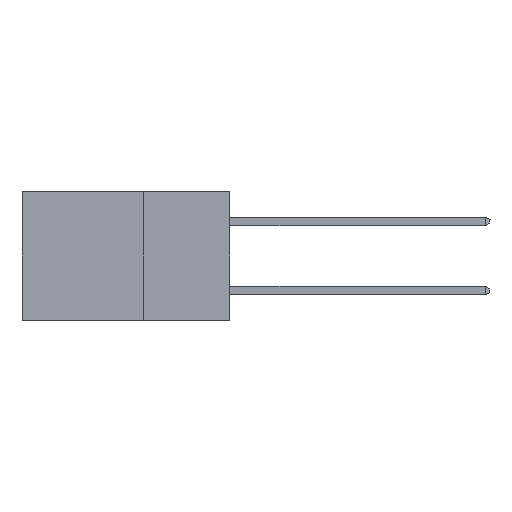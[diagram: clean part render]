
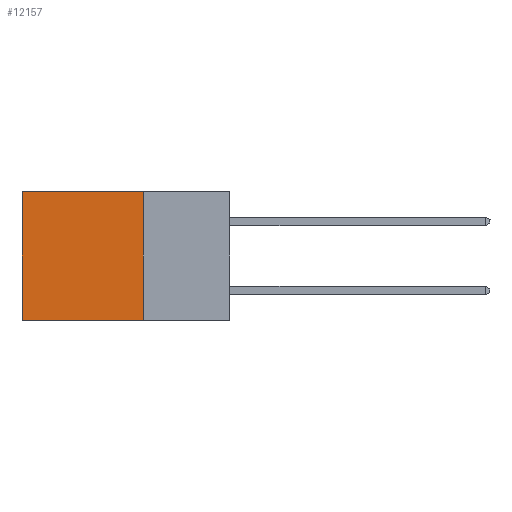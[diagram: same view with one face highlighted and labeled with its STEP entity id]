
A CAD part, left-side view. The second image highlights one B-rep face of the part: STEP entity #12157.
In plain terms, the highlighted planar face has unit normal (-1, 0, 0).
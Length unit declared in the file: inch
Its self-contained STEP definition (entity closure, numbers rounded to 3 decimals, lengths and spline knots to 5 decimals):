
#2193 = FACE_OUTER_BOUND ( 'NONE', #27637, .T. ) ;
#2243 = PLANE ( 'NONE',  #32307 ) ;
#2352 = LINE ( 'NONE', #3856, #28140 ) ;
#2664 = ORIENTED_EDGE ( 'NONE', *, *, #21250, .T. ) ;
#3313 = CARTESIAN_POINT ( 'NONE',  ( 0.298, 0.25, 0. ) ) ;
#3856 = CARTESIAN_POINT ( 'NONE',  ( 0.298, 0.25, 0. ) ) ;
#5920 = LINE ( 'NONE', #29463, #21591 ) ;
#7226 = CARTESIAN_POINT ( 'NONE',  ( 0.298, 0.25, -0.37 ) ) ;
#7919 = EDGE_CURVE ( 'NONE', #17606, #12598, #22392, .T. ) ;
#9897 = EDGE_CURVE ( 'NONE', #25952, #10006, #29351, .T. ) ;
#9940 = EDGE_CURVE ( 'NONE', #25952, #17606, #2352, .T. ) ;
#10006 = VERTEX_POINT ( 'NONE', #13774 ) ;
#12157 = ADVANCED_FACE ( 'NONE', ( #2193 ), #2243, .F. ) ;
#12348 = DIRECTION ( 'NONE',  ( 0., 0., -1. ) ) ;
#12598 = VERTEX_POINT ( 'NONE', #27733 ) ;
#13774 = CARTESIAN_POINT ( 'NONE',  ( 0.298, 0.6, 0. ) ) ;
#14659 = ORIENTED_EDGE ( 'NONE', *, *, #9940, .F. ) ;
#15110 = ORIENTED_EDGE ( 'NONE', *, *, #9897, .T. ) ;
#15202 = VECTOR ( 'NONE', #20756, 39.37008 ) ;
#15276 = VECTOR ( 'NONE', #24626, 39.37008 ) ;
#16486 = CARTESIAN_POINT ( 'NONE',  ( 0.298, 0.25, 0. ) ) ;
#16959 = DIRECTION ( 'NONE',  ( 0., 0., -1. ) ) ;
#17606 = VERTEX_POINT ( 'NONE', #31933 ) ;
#18681 = DIRECTION ( 'NONE',  ( 0., 0., -1. ) ) ;
#20756 = DIRECTION ( 'NONE',  ( 0., 1., 0. ) ) ;
#21250 = EDGE_CURVE ( 'NONE', #10006, #12598, #5920, .T. ) ;
#21591 = VECTOR ( 'NONE', #16959, 39.37008 ) ;
#22392 = LINE ( 'NONE', #7226, #15276 ) ;
#24626 = DIRECTION ( 'NONE',  ( 0., 1., 0. ) ) ;
#25952 = VERTEX_POINT ( 'NONE', #16486 ) ;
#27467 = DIRECTION ( 'NONE',  ( 1., 0., 0. ) ) ;
#27637 = EDGE_LOOP ( 'NONE', ( #2664, #30684, #14659, #15110 ) ) ;
#27733 = CARTESIAN_POINT ( 'NONE',  ( 0.298, 0.6, -0.37 ) ) ;
#28140 = VECTOR ( 'NONE', #18681, 39.37008 ) ;
#29351 = LINE ( 'NONE', #3313, #15202 ) ;
#29463 = CARTESIAN_POINT ( 'NONE',  ( 0.298, 0.6, 0. ) ) ;
#30684 = ORIENTED_EDGE ( 'NONE', *, *, #7919, .F. ) ;
#31933 = CARTESIAN_POINT ( 'NONE',  ( 0.298, 0.25, -0.37 ) ) ;
#32237 = CARTESIAN_POINT ( 'NONE',  ( 0.298, 0.25, 0. ) ) ;
#32307 = AXIS2_PLACEMENT_3D ( 'NONE', #32237, #27467, #12348 ) ;
